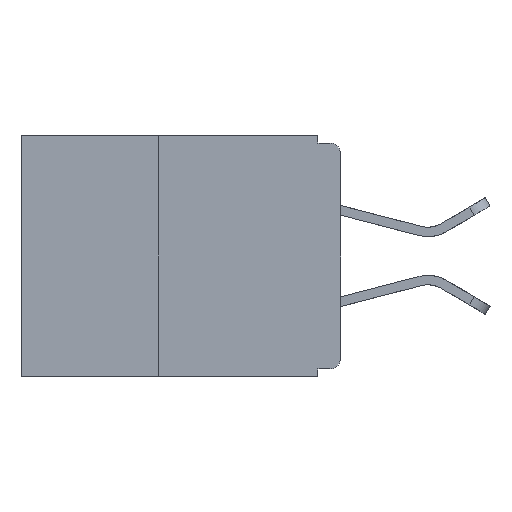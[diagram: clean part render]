
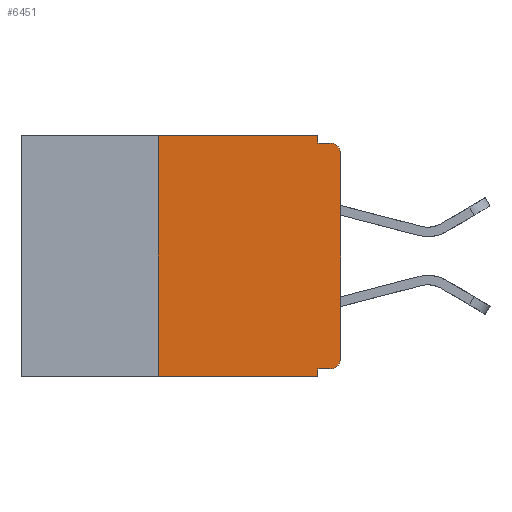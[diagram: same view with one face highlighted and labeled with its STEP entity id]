
A CAD part, left-side view. The second image highlights one B-rep face of the part: STEP entity #6451.
In plain terms, the highlighted planar face has unit normal (-1, 0, 0).
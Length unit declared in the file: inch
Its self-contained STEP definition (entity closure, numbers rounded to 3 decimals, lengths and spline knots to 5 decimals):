
#97 = VERTEX_POINT ( 'NONE', #22398 ) ;
#623 = VECTOR ( 'NONE', #19513, 39.37008 ) ;
#1174 = VECTOR ( 'NONE', #21562, 39.37008 ) ;
#1407 = CARTESIAN_POINT ( 'NONE',  ( 0., 0., -0.305 ) ) ;
#1889 = EDGE_CURVE ( 'NONE', #18422, #21821, #22346, .T. ) ;
#2289 = CARTESIAN_POINT ( 'NONE',  ( 0., 0.437, 0. ) ) ;
#3882 = VERTEX_POINT ( 'NONE', #11424 ) ;
#4398 = FACE_OUTER_BOUND ( 'NONE', #14643, .T. ) ;
#5456 = EDGE_CURVE ( 'NONE', #30879, #21821, #6616, .T. ) ;
#5625 = LINE ( 'NONE', #10379, #26579 ) ;
#6187 = CARTESIAN_POINT ( 'NONE',  ( 0., 0., -0.01 ) ) ;
#6451 = ADVANCED_FACE ( 'NONE', ( #4398 ), #34590, .F. ) ;
#6616 = CIRCLE ( 'NONE', #21269, 0.015 ) ;
#7060 = CARTESIAN_POINT ( 'NONE',  ( 0., 0.015, -0.305 ) ) ;
#7577 = DIRECTION ( 'NONE',  ( 0., 0., 1. ) ) ;
#8164 = CARTESIAN_POINT ( 'NONE',  ( 0., 0.25, -0.33 ) ) ;
#8468 = CARTESIAN_POINT ( 'NONE',  ( 0., 0.015, -0.32 ) ) ;
#8554 = CARTESIAN_POINT ( 'NONE',  ( 0., 0.25, -0.33 ) ) ;
#8665 = VECTOR ( 'NONE', #24210, 39.37008 ) ;
#9396 = VECTOR ( 'NONE', #13725, 39.37008 ) ;
#9552 = CIRCLE ( 'NONE', #23597, 0.015 ) ;
#9863 = DIRECTION ( 'NONE',  ( 0., 0., -1. ) ) ;
#10268 = ORIENTED_EDGE ( 'NONE', *, *, #32247, .F. ) ;
#10379 = CARTESIAN_POINT ( 'NONE',  ( 0., 0., 0. ) ) ;
#10598 = DIRECTION ( 'NONE',  ( -1., 0., 0. ) ) ;
#10952 = DIRECTION ( 'NONE',  ( 0., 0., -1. ) ) ;
#11109 = CARTESIAN_POINT ( 'NONE',  ( 0., 0.015, -0.025 ) ) ;
#11424 = CARTESIAN_POINT ( 'NONE',  ( 0., 0.25, 0. ) ) ;
#11449 = EDGE_CURVE ( 'NONE', #34526, #97, #33541, .T. ) ;
#12515 = CARTESIAN_POINT ( 'NONE',  ( 0., 0.437, -0.33 ) ) ;
#12994 = VECTOR ( 'NONE', #17036, 39.37008 ) ;
#13014 = CARTESIAN_POINT ( 'NONE',  ( 0., 0.015, -0.01 ) ) ;
#13725 = DIRECTION ( 'NONE',  ( 0., 0., -1. ) ) ;
#13761 = ORIENTED_EDGE ( 'NONE', *, *, #18121, .T. ) ;
#14198 = ORIENTED_EDGE ( 'NONE', *, *, #30540, .T. ) ;
#14371 = EDGE_CURVE ( 'NONE', #31548, #3882, #17171, .T. ) ;
#14629 = LINE ( 'NONE', #24895, #20998 ) ;
#14643 = EDGE_LOOP ( 'NONE', ( #14198, #22216, #15907, #10268, #17665, #33455, #13761, #35041, #22660, #23492 ) ) ;
#14961 = EDGE_CURVE ( 'NONE', #97, #27761, #23877, .T. ) ;
#15907 = ORIENTED_EDGE ( 'NONE', *, *, #1889, .F. ) ;
#15973 = LINE ( 'NONE', #2289, #1174 ) ;
#16494 = CARTESIAN_POINT ( 'NONE',  ( 0., 0.031, -0.01 ) ) ;
#17036 = DIRECTION ( 'NONE',  ( 0., 1., 0. ) ) ;
#17171 = LINE ( 'NONE', #8554, #623 ) ;
#17665 = ORIENTED_EDGE ( 'NONE', *, *, #33334, .F. ) ;
#18121 = EDGE_CURVE ( 'NONE', #31548, #27761, #23298, .T. ) ;
#18422 = VERTEX_POINT ( 'NONE', #16494 ) ;
#19390 = EDGE_CURVE ( 'NONE', #34526, #22290, #9552, .T. ) ;
#19513 = DIRECTION ( 'NONE',  ( 0., 0., 1. ) ) ;
#20998 = VECTOR ( 'NONE', #32885, 39.37008 ) ;
#21269 = AXIS2_PLACEMENT_3D ( 'NONE', #11109, #10598, #10952 ) ;
#21288 = CARTESIAN_POINT ( 'NONE',  ( 0., 0.031, 0. ) ) ;
#21562 = DIRECTION ( 'NONE',  ( 0., -1., 0. ) ) ;
#21821 = VERTEX_POINT ( 'NONE', #13014 ) ;
#22216 = ORIENTED_EDGE ( 'NONE', *, *, #5456, .T. ) ;
#22290 = VERTEX_POINT ( 'NONE', #1407 ) ;
#22346 = LINE ( 'NONE', #6187, #8665 ) ;
#22398 = CARTESIAN_POINT ( 'NONE',  ( 0., 0.031, -0.32 ) ) ;
#22660 = ORIENTED_EDGE ( 'NONE', *, *, #11449, .F. ) ;
#23298 = LINE ( 'NONE', #12515, #29544 ) ;
#23492 = ORIENTED_EDGE ( 'NONE', *, *, #19390, .T. ) ;
#23597 = AXIS2_PLACEMENT_3D ( 'NONE', #7060, #26160, #9863 ) ;
#23877 = LINE ( 'NONE', #24693, #9396 ) ;
#24210 = DIRECTION ( 'NONE',  ( 0., -1., 0. ) ) ;
#24693 = CARTESIAN_POINT ( 'NONE',  ( 0., 0.031, -0.33 ) ) ;
#24895 = CARTESIAN_POINT ( 'NONE',  ( 0., 0.031, 0. ) ) ;
#25334 = CARTESIAN_POINT ( 'NONE',  ( 0., 0., -0.025 ) ) ;
#26160 = DIRECTION ( 'NONE',  ( -1., 0., 0. ) ) ;
#26452 = AXIS2_PLACEMENT_3D ( 'NONE', #34508, #34337, #34299 ) ;
#26579 = VECTOR ( 'NONE', #7577, 39.37008 ) ;
#27761 = VERTEX_POINT ( 'NONE', #32999 ) ;
#29544 = VECTOR ( 'NONE', #31328, 39.37008 ) ;
#30540 = EDGE_CURVE ( 'NONE', #22290, #30879, #5625, .T. ) ;
#30879 = VERTEX_POINT ( 'NONE', #25334 ) ;
#31328 = DIRECTION ( 'NONE',  ( 0., -1., 0. ) ) ;
#31548 = VERTEX_POINT ( 'NONE', #8164 ) ;
#32247 = EDGE_CURVE ( 'NONE', #34353, #18422, #14629, .T. ) ;
#32885 = DIRECTION ( 'NONE',  ( 0., 0., -1. ) ) ;
#32982 = CARTESIAN_POINT ( 'NONE',  ( 0., 0., -0.32 ) ) ;
#32999 = CARTESIAN_POINT ( 'NONE',  ( 0., 0.031, -0.33 ) ) ;
#33334 = EDGE_CURVE ( 'NONE', #3882, #34353, #15973, .T. ) ;
#33455 = ORIENTED_EDGE ( 'NONE', *, *, #14371, .F. ) ;
#33541 = LINE ( 'NONE', #32982, #12994 ) ;
#34299 = DIRECTION ( 'NONE',  ( 0., 0., -1. ) ) ;
#34337 = DIRECTION ( 'NONE',  ( 1., 0., 0. ) ) ;
#34353 = VERTEX_POINT ( 'NONE', #21288 ) ;
#34508 = CARTESIAN_POINT ( 'NONE',  ( 0., 0.437, 0. ) ) ;
#34526 = VERTEX_POINT ( 'NONE', #8468 ) ;
#34590 = PLANE ( 'NONE',  #26452 ) ;
#35041 = ORIENTED_EDGE ( 'NONE', *, *, #14961, .F. ) ;
